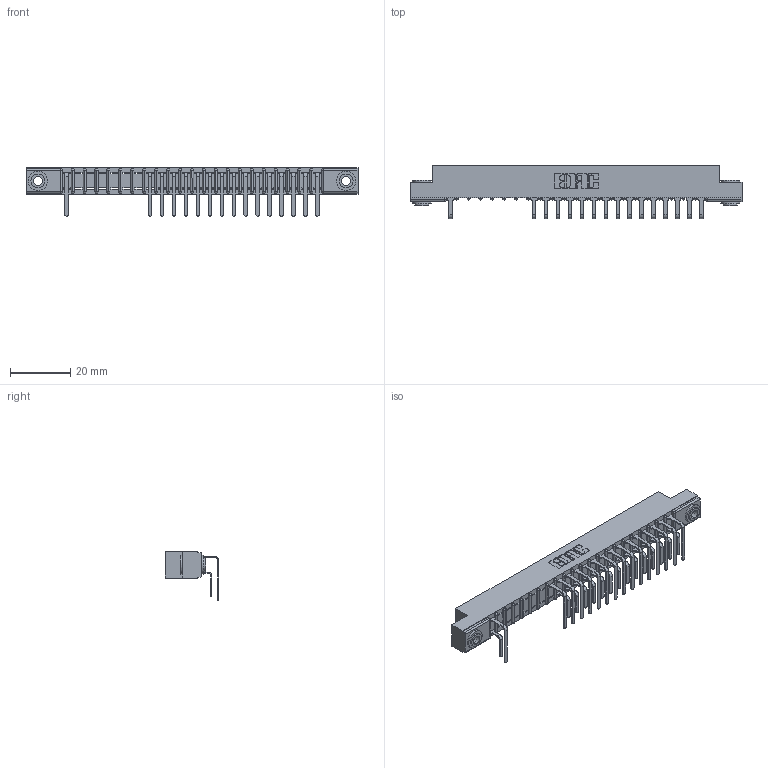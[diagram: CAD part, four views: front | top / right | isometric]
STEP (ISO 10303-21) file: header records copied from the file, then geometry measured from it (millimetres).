
FILE_DESCRIPTION (( 'STEP AP203' ), '1' );
FILE_NAME ('307-022-559-103.STEP', '2018-08-04T03:31:12', ( '' ), ( '' ), 'SwSTEP 2.0', 'SolidWorks 2016', '' );
FILE_SCHEMA (( 'CONFIG_CONTROL_DESIGN' ));
Length unit declared in the file: inch
Products named in the file (5): 345-250-002_345-250-002-102; 307-022-559-103; 307 Part_.156 Dia Mounting Holes; 307-290-001_558 559 - 1 (Single); 307-290-001_559 - 2 (Single)
Assembly tree (34 placements, depth 2):
  307-022-559-103
    307 Part_.156 Dia Mounting Holes
    307-290-001_558 559 - 1 (Single)  x15
    307-290-001_559 - 2 (Single)  x16
    345-250-002_345-250-002-102  x2
Bounding box: 110.19 x 17.69 x 16.08 mm (x, y, z)
Volume: 7179.4 mm3; surface area: 12717.4 mm2
Topology: 34 solids, 34 shells, 1873 faces, 5253 edges, 3394 vertices
Faces by surface type: plane 1195, cylinder 624, sphere 46, cone 8
Entity records: 24126 total; most frequent: CARTESIAN_POINT 3992, ORIENTED_EDGE 3958, DIRECTION 3919, EDGE_CURVE 1979, LINE 1501, VECTOR 1501, VERTEX_POINT 1282, AXIS2_PLACEMENT_3D 1209
